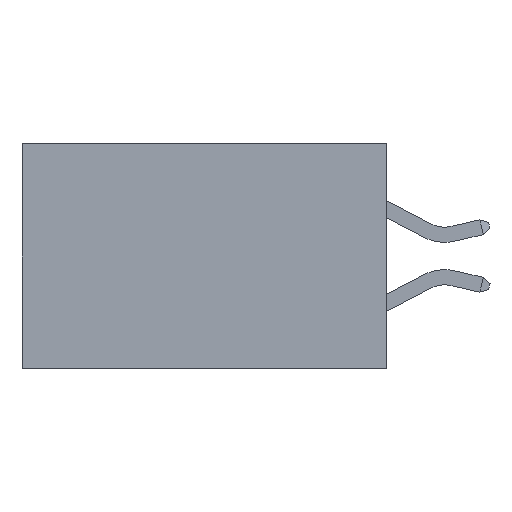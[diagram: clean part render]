
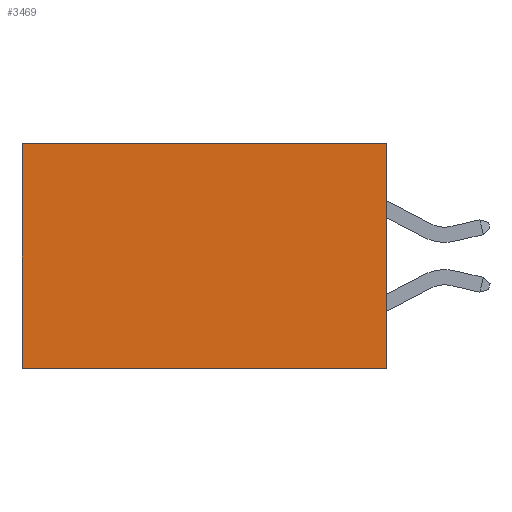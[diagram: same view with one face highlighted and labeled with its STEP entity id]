
A CAD part, left-side view. The second image highlights one B-rep face of the part: STEP entity #3469.
In plain terms, the highlighted planar face has unit normal (-1, 0, 0).
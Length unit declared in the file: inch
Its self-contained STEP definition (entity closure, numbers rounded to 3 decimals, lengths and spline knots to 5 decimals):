
#187 = EDGE_CURVE ( 'NONE', #12278, #4700, #5785, .T. ) ;
#1113 = EDGE_LOOP ( 'NONE', ( #10166, #17514, #10749, #6293 ) ) ;
#1498 = AXIS2_PLACEMENT_3D ( 'NONE', #14334, #13629, #13488 ) ;
#2591 = VECTOR ( 'NONE', #14817, 39.37008 ) ;
#3041 = LINE ( 'NONE', #15033, #2591 ) ;
#3324 = VECTOR ( 'NONE', #14257, 39.37008 ) ;
#3469 = ADVANCED_FACE ( 'NONE', ( #10630 ), #13709, .F. ) ;
#4700 = VERTEX_POINT ( 'NONE', #17159 ) ;
#5785 = LINE ( 'NONE', #13120, #12365 ) ;
#6293 = ORIENTED_EDGE ( 'NONE', *, *, #8769, .T. ) ;
#6575 = VECTOR ( 'NONE', #8788, 39.37008 ) ;
#8376 = CARTESIAN_POINT ( 'NONE',  ( 0.2615, 0., -0.37 ) ) ;
#8769 = EDGE_CURVE ( 'NONE', #11858, #12278, #14587, .T. ) ;
#8788 = DIRECTION ( 'NONE',  ( 0., 0., -1. ) ) ;
#9131 = CARTESIAN_POINT ( 'NONE',  ( 0.2615, 0., -0.37 ) ) ;
#9810 = EDGE_CURVE ( 'NONE', #14464, #4700, #3041, .T. ) ;
#10166 = ORIENTED_EDGE ( 'NONE', *, *, #187, .T. ) ;
#10630 = FACE_OUTER_BOUND ( 'NONE', #1113, .T. ) ;
#10749 = ORIENTED_EDGE ( 'NONE', *, *, #12017, .F. ) ;
#11858 = VERTEX_POINT ( 'NONE', #17694 ) ;
#11883 = CARTESIAN_POINT ( 'NONE',  ( 0.2615, 0.6, 0. ) ) ;
#12017 = EDGE_CURVE ( 'NONE', #11858, #14464, #14023, .T. ) ;
#12278 = VERTEX_POINT ( 'NONE', #11883 ) ;
#12365 = VECTOR ( 'NONE', #16504, 39.37008 ) ;
#13120 = CARTESIAN_POINT ( 'NONE',  ( 0.2615, 0.6, -0.37 ) ) ;
#13488 = DIRECTION ( 'NONE',  ( 0., 0., -1. ) ) ;
#13629 = DIRECTION ( 'NONE',  ( 1., 0., 0. ) ) ;
#13709 = PLANE ( 'NONE',  #1498 ) ;
#14023 = LINE ( 'NONE', #9131, #6575 ) ;
#14257 = DIRECTION ( 'NONE',  ( 0., 1., 0. ) ) ;
#14323 = CARTESIAN_POINT ( 'NONE',  ( 0.2615, 0., 0. ) ) ;
#14334 = CARTESIAN_POINT ( 'NONE',  ( 0.2615, 0., -0.37 ) ) ;
#14464 = VERTEX_POINT ( 'NONE', #8376 ) ;
#14587 = LINE ( 'NONE', #14323, #3324 ) ;
#14817 = DIRECTION ( 'NONE',  ( 0., 1., 0. ) ) ;
#15033 = CARTESIAN_POINT ( 'NONE',  ( 0.2615, 0., -0.37 ) ) ;
#16504 = DIRECTION ( 'NONE',  ( 0., 0., -1. ) ) ;
#17159 = CARTESIAN_POINT ( 'NONE',  ( 0.2615, 0.6, -0.37 ) ) ;
#17514 = ORIENTED_EDGE ( 'NONE', *, *, #9810, .F. ) ;
#17694 = CARTESIAN_POINT ( 'NONE',  ( 0.2615, 0., 0. ) ) ;
